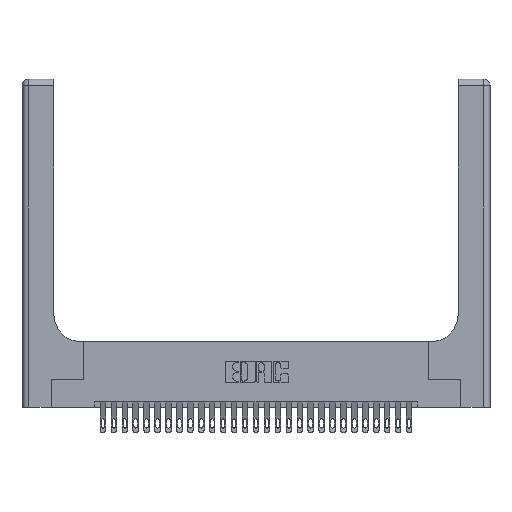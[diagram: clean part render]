
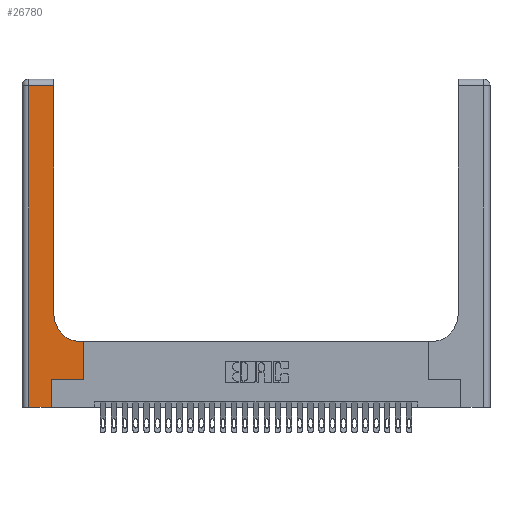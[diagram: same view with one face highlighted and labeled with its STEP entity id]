
A CAD part, top view. The second image highlights one B-rep face of the part: STEP entity #26780.
In plain terms, the highlighted planar face has unit normal (0, 0, 1).
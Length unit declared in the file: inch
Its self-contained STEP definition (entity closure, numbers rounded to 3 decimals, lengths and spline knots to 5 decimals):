
#165 = VECTOR ( 'NONE', #18430, 39.37008 ) ;
#321 = EDGE_CURVE ( 'NONE', #29688, #2976, #24409, .T. ) ;
#338 = VERTEX_POINT ( 'NONE', #15985 ) ;
#551 = CARTESIAN_POINT ( 'NONE',  ( 0., 3., 0.37 ) ) ;
#879 = CARTESIAN_POINT ( 'NONE',  ( 0.2915, 0.6, 0.37 ) ) ;
#1176 = VECTOR ( 'NONE', #18884, 39.37008 ) ;
#1187 = EDGE_CURVE ( 'NONE', #22299, #7728, #20401, .T. ) ;
#1377 = VECTOR ( 'NONE', #6756, 39.37008 ) ;
#1625 = ORIENTED_EDGE ( 'NONE', *, *, #27129, .T. ) ;
#1678 = ORIENTED_EDGE ( 'NONE', *, *, #321, .T. ) ;
#1743 = VERTEX_POINT ( 'NONE', #4710 ) ;
#2037 = ORIENTED_EDGE ( 'NONE', *, *, #6995, .T. ) ;
#2550 = CARTESIAN_POINT ( 'NONE',  ( 0.2915, 0.85, 0.37 ) ) ;
#2941 = VECTOR ( 'NONE', #12105, 39.37008 ) ;
#2976 = VERTEX_POINT ( 'NONE', #17563 ) ;
#3053 = CARTESIAN_POINT ( 'NONE',  ( 0.5585, 0.6, 0.37 ) ) ;
#3781 = EDGE_CURVE ( 'NONE', #7728, #29688, #7112, .T. ) ;
#4710 = CARTESIAN_POINT ( 'NONE',  ( 0.5585, 0.25, 0.37 ) ) ;
#4845 = ORIENTED_EDGE ( 'NONE', *, *, #19364, .T. ) ;
#4952 = CARTESIAN_POINT ( 'NONE',  ( 0., 0., 0.37 ) ) ;
#6756 = DIRECTION ( 'NONE',  ( 0., 1., 0. ) ) ;
#6995 = EDGE_CURVE ( 'NONE', #1743, #16864, #16798, .T. ) ;
#7112 = LINE ( 'NONE', #16103, #165 ) ;
#7278 = DIRECTION ( 'NONE',  ( 0., 0., -1. ) ) ;
#7597 = PLANE ( 'NONE',  #20440 ) ;
#7728 = VERTEX_POINT ( 'NONE', #2550 ) ;
#7775 = ORIENTED_EDGE ( 'NONE', *, *, #3781, .T. ) ;
#8954 = DIRECTION ( 'NONE',  ( 0., 1., 0. ) ) ;
#9768 = CARTESIAN_POINT ( 'NONE',  ( 0.06, 3., 0.37 ) ) ;
#9822 = DIRECTION ( 'NONE',  ( 1., 0., 0. ) ) ;
#9971 = DIRECTION ( 'NONE',  ( -1., 0., 0. ) ) ;
#10149 = ORIENTED_EDGE ( 'NONE', *, *, #25139, .T. ) ;
#10216 = VECTOR ( 'NONE', #19499, 39.37008 ) ;
#10461 = CARTESIAN_POINT ( 'NONE',  ( 0.06, 0., 0.37 ) ) ;
#10646 = VECTOR ( 'NONE', #8954, 39.37008 ) ;
#12105 = DIRECTION ( 'NONE',  ( 0., -1., 0. ) ) ;
#12342 = LINE ( 'NONE', #20652, #1377 ) ;
#13043 = VERTEX_POINT ( 'NONE', #10461 ) ;
#14277 = EDGE_LOOP ( 'NONE', ( #7775, #1678, #4845, #17531, #1625, #10149, #2037, #15290, #26514 ) ) ;
#15290 = ORIENTED_EDGE ( 'NONE', *, *, #26327, .T. ) ;
#15985 = CARTESIAN_POINT ( 'NONE',  ( 0.269, 0., 0.37 ) ) ;
#16103 = CARTESIAN_POINT ( 'NONE',  ( 0.2915, 3., 0.37 ) ) ;
#16108 = LINE ( 'NONE', #9768, #2941 ) ;
#16798 = LINE ( 'NONE', #22769, #10646 ) ;
#16817 = VECTOR ( 'NONE', #9822, 39.37008 ) ;
#16819 = CARTESIAN_POINT ( 'NONE',  ( 0.5415, 0.6, 0.37 ) ) ;
#16864 = VERTEX_POINT ( 'NONE', #3053 ) ;
#17104 = LINE ( 'NONE', #879, #10216 ) ;
#17531 = ORIENTED_EDGE ( 'NONE', *, *, #19166, .T. ) ;
#17563 = CARTESIAN_POINT ( 'NONE',  ( 0.06, 2.94, 0.37 ) ) ;
#18321 = VECTOR ( 'NONE', #20505, 39.37008 ) ;
#18430 = DIRECTION ( 'NONE',  ( 0., 1., 0. ) ) ;
#18884 = DIRECTION ( 'NONE',  ( 1., 0., 0. ) ) ;
#19166 = EDGE_CURVE ( 'NONE', #13043, #338, #25833, .T. ) ;
#19364 = EDGE_CURVE ( 'NONE', #2976, #13043, #16108, .T. ) ;
#19499 = DIRECTION ( 'NONE',  ( -1., 0., 0. ) ) ;
#19937 = VERTEX_POINT ( 'NONE', #23732 ) ;
#20401 = CIRCLE ( 'NONE', #28780, 0.25 ) ;
#20440 = AXIS2_PLACEMENT_3D ( 'NONE', #551, #23785, #9971 ) ;
#20505 = DIRECTION ( 'NONE',  ( -1., 0., 0. ) ) ;
#20652 = CARTESIAN_POINT ( 'NONE',  ( 0.269, 0., 0.37 ) ) ;
#21158 = CARTESIAN_POINT ( 'NONE',  ( 0.5415, 0.85, 0.37 ) ) ;
#21325 = CARTESIAN_POINT ( 'NONE',  ( 0.269, 0.25, 0.37 ) ) ;
#22299 = VERTEX_POINT ( 'NONE', #16819 ) ;
#22436 = FACE_OUTER_BOUND ( 'NONE', #14277, .T. ) ;
#22476 = CARTESIAN_POINT ( 'NONE',  ( 0.2915, 2.94, 0.37 ) ) ;
#22769 = CARTESIAN_POINT ( 'NONE',  ( 0.5585, 0.25, 0.37 ) ) ;
#23482 = DIRECTION ( 'NONE',  ( 1., 0., 0. ) ) ;
#23732 = CARTESIAN_POINT ( 'NONE',  ( 0.269, 0.25, 0.37 ) ) ;
#23785 = DIRECTION ( 'NONE',  ( 0., 0., -1. ) ) ;
#24409 = LINE ( 'NONE', #29654, #18321 ) ;
#25139 = EDGE_CURVE ( 'NONE', #19937, #1743, #29042, .T. ) ;
#25833 = LINE ( 'NONE', #4952, #1176 ) ;
#26327 = EDGE_CURVE ( 'NONE', #16864, #22299, #17104, .T. ) ;
#26514 = ORIENTED_EDGE ( 'NONE', *, *, #1187, .T. ) ;
#26780 = ADVANCED_FACE ( 'NONE', ( #22436 ), #7597, .F. ) ;
#27129 = EDGE_CURVE ( 'NONE', #338, #19937, #12342, .T. ) ;
#28780 = AXIS2_PLACEMENT_3D ( 'NONE', #21158, #7278, #23482 ) ;
#29042 = LINE ( 'NONE', #21325, #16817 ) ;
#29654 = CARTESIAN_POINT ( 'NONE',  ( 0., 2.94, 0.37 ) ) ;
#29688 = VERTEX_POINT ( 'NONE', #22476 ) ;
